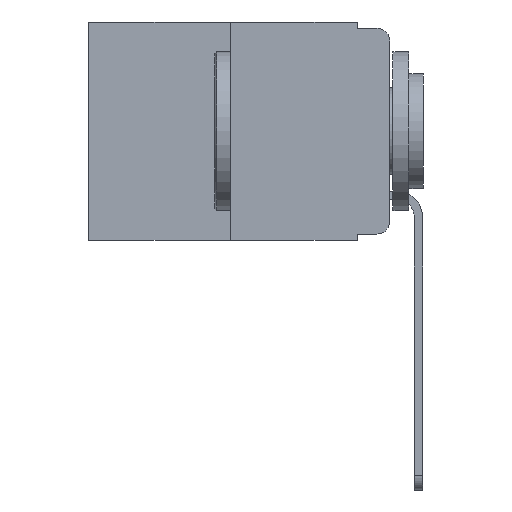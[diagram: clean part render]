
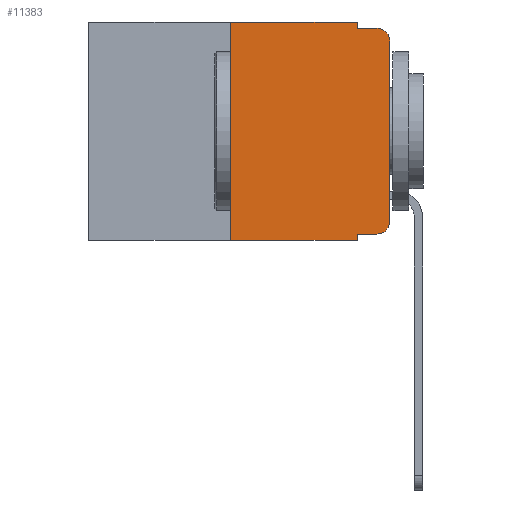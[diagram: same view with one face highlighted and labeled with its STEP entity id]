
A CAD part, left-side view. The second image highlights one B-rep face of the part: STEP entity #11383.
In plain terms, the highlighted planar face has unit normal (-1, 0, 0).
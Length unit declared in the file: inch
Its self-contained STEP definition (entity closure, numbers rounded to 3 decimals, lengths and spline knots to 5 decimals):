
#384 = ORIENTED_EDGE ( 'NONE', *, *, #912, .F. ) ;
#614 = VECTOR ( 'NONE', #15906, 39.37008 ) ;
#685 = VECTOR ( 'NONE', #7877, 39.37008 ) ;
#912 = EDGE_CURVE ( 'NONE', #12136, #3016, #10304, .T. ) ;
#917 = ORIENTED_EDGE ( 'NONE', *, *, #14819, .F. ) ;
#1045 = VERTEX_POINT ( 'NONE', #14121 ) ;
#1074 = CARTESIAN_POINT ( 'NONE',  ( 0., 0.473, -0.343 ) ) ;
#1162 = DIRECTION ( 'NONE',  ( 0., -1., 0. ) ) ;
#1167 = DIRECTION ( 'NONE',  ( -1., 0., 0. ) ) ;
#1178 = ORIENTED_EDGE ( 'NONE', *, *, #13154, .T. ) ;
#1418 = ORIENTED_EDGE ( 'NONE', *, *, #2257, .T. ) ;
#1783 = CARTESIAN_POINT ( 'NONE',  ( 0., 0., -0.313 ) ) ;
#1832 = FACE_OUTER_BOUND ( 'NONE', #10721, .T. ) ;
#1989 = EDGE_CURVE ( 'NONE', #2206, #3016, #10273, .T. ) ;
#2006 = AXIS2_PLACEMENT_3D ( 'NONE', #10633, #15717, #8009 ) ;
#2039 = CARTESIAN_POINT ( 'NONE',  ( 0., 0., 0. ) ) ;
#2206 = VERTEX_POINT ( 'NONE', #2542 ) ;
#2257 = EDGE_CURVE ( 'NONE', #7485, #11483, #10065, .T. ) ;
#2417 = VERTEX_POINT ( 'NONE', #1783 ) ;
#2475 = CARTESIAN_POINT ( 'NONE',  ( 0., 0.25, -0.343 ) ) ;
#2542 = CARTESIAN_POINT ( 'NONE',  ( 0., 0., -0.03 ) ) ;
#3012 = EDGE_CURVE ( 'NONE', #2417, #2206, #11698, .T. ) ;
#3016 = VERTEX_POINT ( 'NONE', #3778 ) ;
#3131 = ORIENTED_EDGE ( 'NONE', *, *, #11422, .T. ) ;
#3778 = CARTESIAN_POINT ( 'NONE',  ( 0., 0.02, -0.01 ) ) ;
#3930 = CARTESIAN_POINT ( 'NONE',  ( 0., 0.051, 0. ) ) ;
#4120 = DIRECTION ( 'NONE',  ( 0., 0., -1. ) ) ;
#4944 = AXIS2_PLACEMENT_3D ( 'NONE', #9497, #1167, #10803 ) ;
#4993 = DIRECTION ( 'NONE',  ( 0., 0., 1. ) ) ;
#5595 = DIRECTION ( 'NONE',  ( 0., 0., 1. ) ) ;
#6114 = AXIS2_PLACEMENT_3D ( 'NONE', #8811, #8792, #8768 ) ;
#6239 = LINE ( 'NONE', #10657, #12855 ) ;
#6765 = VECTOR ( 'NONE', #7016, 39.37008 ) ;
#6893 = CARTESIAN_POINT ( 'NONE',  ( 0., 0.051, -0.343 ) ) ;
#6995 = CARTESIAN_POINT ( 'NONE',  ( 0., 0.051, -0.01 ) ) ;
#7016 = DIRECTION ( 'NONE',  ( 0., -1., 0. ) ) ;
#7485 = VERTEX_POINT ( 'NONE', #2475 ) ;
#7738 = ORIENTED_EDGE ( 'NONE', *, *, #15744, .F. ) ;
#7742 = VECTOR ( 'NONE', #5595, 39.37008 ) ;
#7877 = DIRECTION ( 'NONE',  ( 0., 0., -1. ) ) ;
#8009 = DIRECTION ( 'NONE',  ( 0., 0., -1. ) ) ;
#8039 = VECTOR ( 'NONE', #10066, 39.37008 ) ;
#8340 = VERTEX_POINT ( 'NONE', #8378 ) ;
#8378 = CARTESIAN_POINT ( 'NONE',  ( 0., 0.051, 0. ) ) ;
#8559 = LINE ( 'NONE', #12851, #12486 ) ;
#8768 = DIRECTION ( 'NONE',  ( 0., 0., -1. ) ) ;
#8792 = DIRECTION ( 'NONE',  ( -1., 0., 0. ) ) ;
#8811 = CARTESIAN_POINT ( 'NONE',  ( 0., 0.02, -0.03 ) ) ;
#9036 = LINE ( 'NONE', #3930, #685 ) ;
#9497 = CARTESIAN_POINT ( 'NONE',  ( 0., 0.02, -0.313 ) ) ;
#10065 = LINE ( 'NONE', #1074, #13124 ) ;
#10066 = DIRECTION ( 'NONE',  ( 0., -1., 0. ) ) ;
#10273 = CIRCLE ( 'NONE', #6114, 0.02 ) ;
#10304 = LINE ( 'NONE', #6995, #6765 ) ;
#10633 = CARTESIAN_POINT ( 'NONE',  ( 0., 0.473, 0. ) ) ;
#10657 = CARTESIAN_POINT ( 'NONE',  ( 0., 0.051, 0. ) ) ;
#10721 = EDGE_LOOP ( 'NONE', ( #14438, #12483, #384, #15974, #7738, #917, #1418, #16380, #1178, #3131 ) ) ;
#10803 = DIRECTION ( 'NONE',  ( 0., 0., -1. ) ) ;
#11383 = ADVANCED_FACE ( 'NONE', ( #1832 ), #14503, .F. ) ;
#11391 = CARTESIAN_POINT ( 'NONE',  ( 0., 0.051, -0.333 ) ) ;
#11422 = EDGE_CURVE ( 'NONE', #13937, #2417, #15543, .T. ) ;
#11483 = VERTEX_POINT ( 'NONE', #6893 ) ;
#11698 = LINE ( 'NONE', #2039, #7742 ) ;
#12136 = VERTEX_POINT ( 'NONE', #15911 ) ;
#12483 = ORIENTED_EDGE ( 'NONE', *, *, #1989, .T. ) ;
#12486 = VECTOR ( 'NONE', #4993, 39.37008 ) ;
#12851 = CARTESIAN_POINT ( 'NONE',  ( 0., 0.25, 0. ) ) ;
#12855 = VECTOR ( 'NONE', #4120, 39.37008 ) ;
#13124 = VECTOR ( 'NONE', #1162, 39.37008 ) ;
#13154 = EDGE_CURVE ( 'NONE', #1045, #13937, #14927, .T. ) ;
#13937 = VERTEX_POINT ( 'NONE', #16732 ) ;
#13985 = EDGE_CURVE ( 'NONE', #1045, #11483, #9036, .T. ) ;
#14121 = CARTESIAN_POINT ( 'NONE',  ( 0., 0.051, -0.333 ) ) ;
#14438 = ORIENTED_EDGE ( 'NONE', *, *, #3012, .T. ) ;
#14503 = PLANE ( 'NONE',  #2006 ) ;
#14699 = CARTESIAN_POINT ( 'NONE',  ( 0., 0.473, 0. ) ) ;
#14819 = EDGE_CURVE ( 'NONE', #7485, #15918, #8559, .T. ) ;
#14927 = LINE ( 'NONE', #11391, #8039 ) ;
#14988 = LINE ( 'NONE', #14699, #614 ) ;
#15053 = CARTESIAN_POINT ( 'NONE',  ( 0., 0.25, 0. ) ) ;
#15543 = CIRCLE ( 'NONE', #4944, 0.02 ) ;
#15634 = EDGE_CURVE ( 'NONE', #8340, #12136, #6239, .T. ) ;
#15717 = DIRECTION ( 'NONE',  ( 1., 0., 0. ) ) ;
#15744 = EDGE_CURVE ( 'NONE', #15918, #8340, #14988, .T. ) ;
#15906 = DIRECTION ( 'NONE',  ( 0., -1., 0. ) ) ;
#15911 = CARTESIAN_POINT ( 'NONE',  ( 0., 0.051, -0.01 ) ) ;
#15918 = VERTEX_POINT ( 'NONE', #15053 ) ;
#15974 = ORIENTED_EDGE ( 'NONE', *, *, #15634, .F. ) ;
#16380 = ORIENTED_EDGE ( 'NONE', *, *, #13985, .F. ) ;
#16732 = CARTESIAN_POINT ( 'NONE',  ( 0., 0.02, -0.333 ) ) ;
